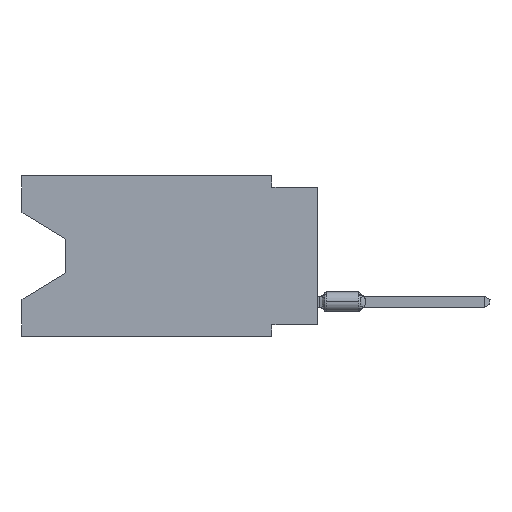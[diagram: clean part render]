
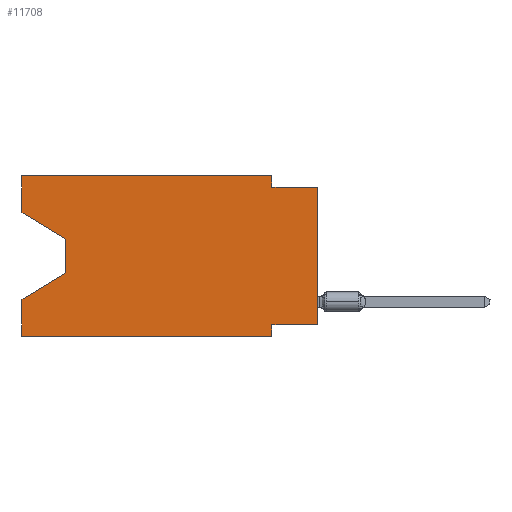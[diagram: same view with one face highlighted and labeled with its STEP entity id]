
A CAD part, left-side view. The second image highlights one B-rep face of the part: STEP entity #11708.
In plain terms, the highlighted planar face has unit normal (-1, 0, 0).
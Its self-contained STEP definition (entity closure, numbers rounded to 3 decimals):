
#537 = VERTEX_POINT ( 'NONE', #8318 ) ;
#1312 = VERTEX_POINT ( 'NONE', #57594 ) ;
#1607 = VERTEX_POINT ( 'NONE', #38262 ) ;
#1959 = PLANE ( 'NONE',  #57395 ) ;
#3026 = FACE_OUTER_BOUND ( 'NONE', #4764, .T. ) ;
#4764 = EDGE_LOOP ( 'NONE', ( #26774, #36877, #86324, #93655, #69164, #44245, #103698, #82796, #41958, #94430, #52809, #93661 ) ) ;
#8318 = CARTESIAN_POINT ( 'NONE',  ( 0., 0., -0.635 ) ) ;
#8866 = VECTOR ( 'NONE', #33872, 1000. ) ;
#9510 = LINE ( 'NONE', #26562, #93043 ) ;
#10739 = CARTESIAN_POINT ( 'NONE',  ( 0., 13.97, -3.505 ) ) ;
#11098 = EDGE_CURVE ( 'NONE', #96127, #18550, #14759, .T. ) ;
#11708 = ADVANCED_FACE ( 'NONE', ( #3026 ), #1959, .F. ) ;
#12459 = VECTOR ( 'NONE', #82743, 1000. ) ;
#13683 = DIRECTION ( 'NONE',  ( 0., -0.855, -0.519 ) ) ;
#14759 = LINE ( 'NONE', #21952, #90670 ) ;
#15418 = CARTESIAN_POINT ( 'NONE',  ( 0., 16.383, -8.89 ) ) ;
#15622 = CARTESIAN_POINT ( 'NONE',  ( 0., 0., 0. ) ) ;
#15704 = VERTEX_POINT ( 'NONE', #40680 ) ;
#16814 = LINE ( 'NONE', #49300, #8866 ) ;
#17439 = LINE ( 'NONE', #41678, #49414 ) ;
#18458 = DIRECTION ( 'NONE',  ( 0., 0., -1. ) ) ;
#18550 = VERTEX_POINT ( 'NONE', #10739 ) ;
#18552 = LINE ( 'NONE', #108773, #32497 ) ;
#21952 = CARTESIAN_POINT ( 'NONE',  ( 0., 16.383, -2.038 ) ) ;
#23761 = CARTESIAN_POINT ( 'NONE',  ( 0., 16.383, -8.89 ) ) ;
#25576 = DIRECTION ( 'NONE',  ( 0., 0., 1. ) ) ;
#25632 = CARTESIAN_POINT ( 'NONE',  ( 0., 13.97, -3.505 ) ) ;
#26562 = CARTESIAN_POINT ( 'NONE',  ( 0., 2.54, -8.89 ) ) ;
#26774 = ORIENTED_EDGE ( 'NONE', *, *, #11098, .T. ) ;
#27268 = LINE ( 'NONE', #25632, #78232 ) ;
#27740 = CARTESIAN_POINT ( 'NONE',  ( 0., 16.383, 0. ) ) ;
#28332 = CARTESIAN_POINT ( 'NONE',  ( 0., 13.97, -5.385 ) ) ;
#30572 = VECTOR ( 'NONE', #53646, 1000. ) ;
#32497 = VECTOR ( 'NONE', #67549, 1000. ) ;
#33872 = DIRECTION ( 'NONE',  ( 0., 1., 0. ) ) ;
#35670 = EDGE_CURVE ( 'NONE', #56030, #100632, #104208, .T. ) ;
#36877 = ORIENTED_EDGE ( 'NONE', *, *, #46863, .T. ) ;
#38262 = CARTESIAN_POINT ( 'NONE',  ( 0., 2.54, -8.255 ) ) ;
#40680 = CARTESIAN_POINT ( 'NONE',  ( 0., 2.54, -8.89 ) ) ;
#41678 = CARTESIAN_POINT ( 'NONE',  ( 0., 0., -0.635 ) ) ;
#41958 = ORIENTED_EDGE ( 'NONE', *, *, #93586, .F. ) ;
#42670 = DIRECTION ( 'NONE',  ( 0., 0., -1. ) ) ;
#43777 = EDGE_CURVE ( 'NONE', #108620, #537, #108554, .T. ) ;
#44245 = ORIENTED_EDGE ( 'NONE', *, *, #71954, .F. ) ;
#44796 = LINE ( 'NONE', #27740, #97600 ) ;
#46863 = EDGE_CURVE ( 'NONE', #18550, #63718, #27268, .T. ) ;
#49300 = CARTESIAN_POINT ( 'NONE',  ( 0., 0., -8.255 ) ) ;
#49414 = VECTOR ( 'NONE', #76850, 1000. ) ;
#51586 = LINE ( 'NONE', #52121, #97149 ) ;
#52121 = CARTESIAN_POINT ( 'NONE',  ( 0., 16.383, 0. ) ) ;
#52637 = VERTEX_POINT ( 'NONE', #79329 ) ;
#52809 = ORIENTED_EDGE ( 'NONE', *, *, #35670, .F. ) ;
#53646 = DIRECTION ( 'NONE',  ( 0., -1., 0. ) ) ;
#54811 = EDGE_CURVE ( 'NONE', #108620, #1607, #16814, .T. ) ;
#55481 = CARTESIAN_POINT ( 'NONE',  ( 0., 0., -8.255 ) ) ;
#56030 = VERTEX_POINT ( 'NONE', #75704 ) ;
#57395 = AXIS2_PLACEMENT_3D ( 'NONE', #59180, #67974, #42670 ) ;
#57594 = CARTESIAN_POINT ( 'NONE',  ( 0., 16.383, -6.852 ) ) ;
#58318 = EDGE_CURVE ( 'NONE', #69444, #1312, #44796, .T. ) ;
#58894 = CARTESIAN_POINT ( 'NONE',  ( 0., 16.383, -2.038 ) ) ;
#59180 = CARTESIAN_POINT ( 'NONE',  ( 0., 16.383, 0. ) ) ;
#62427 = DIRECTION ( 'NONE',  ( 0., 0.855, -0.519 ) ) ;
#63718 = VERTEX_POINT ( 'NONE', #106244 ) ;
#66689 = LINE ( 'NONE', #23761, #94993 ) ;
#67549 = DIRECTION ( 'NONE',  ( 0., 0., -1. ) ) ;
#67974 = DIRECTION ( 'NONE',  ( 1., 0., 0. ) ) ;
#69164 = ORIENTED_EDGE ( 'NONE', *, *, #74346, .T. ) ;
#69444 = VERTEX_POINT ( 'NONE', #15418 ) ;
#69939 = EDGE_CURVE ( 'NONE', #100632, #52637, #18552, .T. ) ;
#70155 = LINE ( 'NONE', #28332, #80888 ) ;
#71954 = EDGE_CURVE ( 'NONE', #1607, #15704, #9510, .T. ) ;
#72926 = EDGE_CURVE ( 'NONE', #63718, #1312, #70155, .T. ) ;
#74346 = EDGE_CURVE ( 'NONE', #69444, #15704, #66689, .T. ) ;
#75704 = CARTESIAN_POINT ( 'NONE',  ( 0., 16.383, 0. ) ) ;
#75811 = DIRECTION ( 'NONE',  ( 0., 0., 1. ) ) ;
#76850 = DIRECTION ( 'NONE',  ( 0., -1., 0. ) ) ;
#78232 = VECTOR ( 'NONE', #18458, 1000. ) ;
#78946 = CARTESIAN_POINT ( 'NONE',  ( 0., 16.383, 0. ) ) ;
#79329 = CARTESIAN_POINT ( 'NONE',  ( 0., 2.54, -0.635 ) ) ;
#80888 = VECTOR ( 'NONE', #62427, 1000. ) ;
#82743 = DIRECTION ( 'NONE',  ( 0., 0., 1. ) ) ;
#82796 = ORIENTED_EDGE ( 'NONE', *, *, #43777, .T. ) ;
#82988 = EDGE_CURVE ( 'NONE', #96127, #56030, #51586, .T. ) ;
#86324 = ORIENTED_EDGE ( 'NONE', *, *, #72926, .T. ) ;
#90670 = VECTOR ( 'NONE', #13683, 1000. ) ;
#93043 = VECTOR ( 'NONE', #100282, 1000. ) ;
#93586 = EDGE_CURVE ( 'NONE', #52637, #537, #17439, .T. ) ;
#93655 = ORIENTED_EDGE ( 'NONE', *, *, #58318, .F. ) ;
#93661 = ORIENTED_EDGE ( 'NONE', *, *, #82988, .F. ) ;
#94430 = ORIENTED_EDGE ( 'NONE', *, *, #69939, .F. ) ;
#94448 = CARTESIAN_POINT ( 'NONE',  ( 0., 2.54, 0. ) ) ;
#94993 = VECTOR ( 'NONE', #107909, 1000. ) ;
#96127 = VERTEX_POINT ( 'NONE', #58894 ) ;
#97149 = VECTOR ( 'NONE', #75811, 1000. ) ;
#97600 = VECTOR ( 'NONE', #25576, 1000. ) ;
#100282 = DIRECTION ( 'NONE',  ( 0., 0., -1. ) ) ;
#100632 = VERTEX_POINT ( 'NONE', #94448 ) ;
#103698 = ORIENTED_EDGE ( 'NONE', *, *, #54811, .F. ) ;
#104208 = LINE ( 'NONE', #78946, #30572 ) ;
#106244 = CARTESIAN_POINT ( 'NONE',  ( 0., 13.97, -5.385 ) ) ;
#107909 = DIRECTION ( 'NONE',  ( 0., -1., 0. ) ) ;
#108554 = LINE ( 'NONE', #15622, #12459 ) ;
#108620 = VERTEX_POINT ( 'NONE', #55481 ) ;
#108773 = CARTESIAN_POINT ( 'NONE',  ( 0., 2.54, 0. ) ) ;
